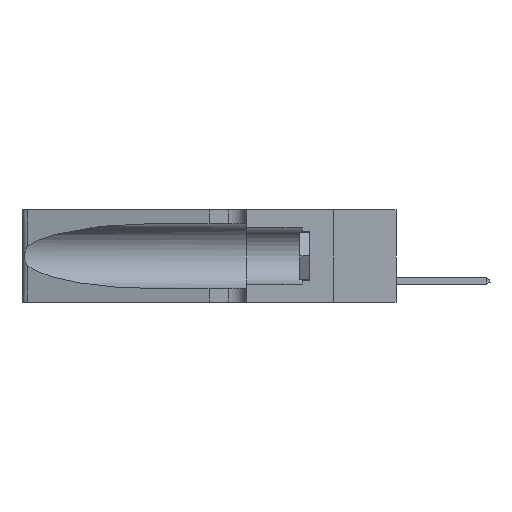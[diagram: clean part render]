
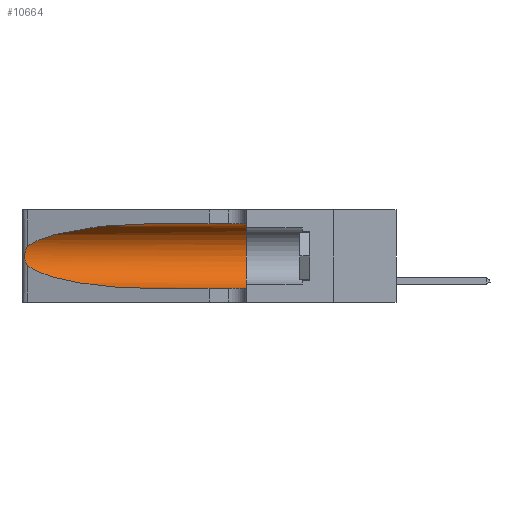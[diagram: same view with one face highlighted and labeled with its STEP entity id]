
A CAD part, left-side view. The second image highlights one B-rep face of the part: STEP entity #10664.
In plain terms, the highlighted cylindrical face has radius 3.308 mm (diameter 6.617 mm), a partial arc.
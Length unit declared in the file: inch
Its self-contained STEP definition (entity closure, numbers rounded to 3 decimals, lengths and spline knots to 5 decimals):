
#4 = CARTESIAN_POINT ( 'NONE',  ( 0.1305, 0.35, 0.31525 ) ) ;
#23 = ORIENTED_EDGE ( 'NONE', *, *, #19158, .F. ) ;
#494 = CARTESIAN_POINT ( 'NONE',  ( 0.25555, 1.22993, 0.14849 ) ) ;
#728 = CARTESIAN_POINT ( 'NONE',  ( 0.18966, 0.96281, 0.05475 ) ) ;
#735 = CARTESIAN_POINT ( 'NONE',  ( 0.25487, 1.22718, 0.22369 ) ) ;
#1291 = DIRECTION ( 'NONE',  ( 0., -1., 0. ) ) ;
#1367 = AXIS2_PLACEMENT_3D ( 'NONE', #32556, #1291, #26429 ) ;
#1654 = LINE ( 'NONE', #19210, #11016 ) ;
#2381 = DIRECTION ( 'NONE',  ( 0., 1., 0. ) ) ;
#3594 =( BOUNDED_CURVE ( )  B_SPLINE_CURVE ( 3, ( #3757, #31983, #19567, #735 ),
 .UNSPECIFIED., .F., .F. ) 
 B_SPLINE_CURVE_WITH_KNOTS ( ( 4, 4 ),
 ( 1.5708, 2.84003 ),
 .UNSPECIFIED. ) 
 CURVE ( )  GEOMETRIC_REPRESENTATION_ITEM ( )  RATIONAL_B_SPLINE_CURVE ( ( 1., 0.87, 0.87, 1. ) ) 
 REPRESENTATION_ITEM ( '' )  );
#3757 = CARTESIAN_POINT ( 'NONE',  ( 0.1305, 0.72297, 0.31525 ) ) ;
#5365 = CARTESIAN_POINT ( 'NONE',  ( 0.26075, 1.23896, 0.19203 ) ) ;
#5766 = CARTESIAN_POINT ( 'NONE',  ( 0.26017, 1.23833, 0.17102 ) ) ;
#6132 = B_SPLINE_CURVE_WITH_KNOTS ( 'NONE', 3,
 ( #21737, #19653, #10298, #34682, #15936, #33316, #5365, #36600, #5766, #25374, #19859, #9836, #494, #10801 ),
 .UNSPECIFIED., .F., .F.,
 ( 4, 2, 2, 2, 2, 2, 4 ),
 ( 0., 0.00027, 0.00053, 0.00107, 0.0016, 0.00187, 0.00214 ),
 .UNSPECIFIED. ) ;
#6806 = CARTESIAN_POINT ( 'NONE',  ( 0.1305, 0.72297, 0.31525 ) ) ;
#6896 = CARTESIAN_POINT ( 'NONE',  ( 0.2373, 1.15595, 0.08982 ) ) ;
#7264 = CARTESIAN_POINT ( 'NONE',  ( 0.25487, 1.22718, 0.14631 ) ) ;
#8649 =( BOUNDED_CURVE ( )  B_SPLINE_CURVE ( 3, ( #38559, #6896, #728, #13506 ),
 .UNSPECIFIED., .F., .T. ) 
 B_SPLINE_CURVE_WITH_KNOTS ( ( 4, 4 ),
 ( 3.44316, 4.71239 ),
 .UNSPECIFIED. ) 
 CURVE ( )  GEOMETRIC_REPRESENTATION_ITEM ( )  RATIONAL_B_SPLINE_CURVE ( ( 1., 0.87, 0.87, 1. ) ) 
 REPRESENTATION_ITEM ( '' )  );
#9836 = CARTESIAN_POINT ( 'NONE',  ( 0.25639, 1.23186, 0.15144 ) ) ;
#10298 = CARTESIAN_POINT ( 'NONE',  ( 0.25639, 1.23184, 0.21858 ) ) ;
#10318 = EDGE_CURVE ( 'NONE', #38061, #22144, #28566, .T. ) ;
#10664 = ADVANCED_FACE ( 'NONE', ( #22173 ), #20757, .F. ) ;
#10801 = CARTESIAN_POINT ( 'NONE',  ( 0.25487, 1.22718, 0.14631 ) ) ;
#11016 = VECTOR ( 'NONE', #28136, 39.37008 ) ;
#12293 = DIRECTION ( 'NONE',  ( 0., -1., 0. ) ) ;
#13506 = CARTESIAN_POINT ( 'NONE',  ( 0.1305, 0.72297, 0.05475 ) ) ;
#15395 = VERTEX_POINT ( 'NONE', #31960 ) ;
#15936 = CARTESIAN_POINT ( 'NONE',  ( 0.25854, 1.2359, 0.20912 ) ) ;
#18486 = VERTEX_POINT ( 'NONE', #24417 ) ;
#19158 = EDGE_CURVE ( 'NONE', #23002, #38061, #21104, .T. ) ;
#19210 = CARTESIAN_POINT ( 'NONE',  ( 0.1305, 1.61858, 0.05475 ) ) ;
#19511 = VERTEX_POINT ( 'NONE', #7264 ) ;
#19567 = CARTESIAN_POINT ( 'NONE',  ( 0.2373, 1.15595, 0.28018 ) ) ;
#19653 = CARTESIAN_POINT ( 'NONE',  ( 0.25555, 1.22994, 0.2215 ) ) ;
#19859 = CARTESIAN_POINT ( 'NONE',  ( 0.25789, 1.23486, 0.15765 ) ) ;
#20037 = CARTESIAN_POINT ( 'NONE',  ( 0.1305, 0.35, 0.05475 ) ) ;
#20651 = EDGE_CURVE ( 'NONE', #19511, #15395, #8649, .T. ) ;
#20757 = CYLINDRICAL_SURFACE ( 'NONE', #1367, 0.13025 ) ;
#21104 = LINE ( 'NONE', #24922, #38686 ) ;
#21737 = CARTESIAN_POINT ( 'NONE',  ( 0.25487, 1.22718, 0.22369 ) ) ;
#22144 = VERTEX_POINT ( 'NONE', #20037 ) ;
#22173 = FACE_OUTER_BOUND ( 'NONE', #33505, .T. ) ;
#23002 = VERTEX_POINT ( 'NONE', #6806 ) ;
#23127 = ORIENTED_EDGE ( 'NONE', *, *, #25443, .T. ) ;
#24417 = CARTESIAN_POINT ( 'NONE',  ( 0.25487, 1.22718, 0.22369 ) ) ;
#24922 = CARTESIAN_POINT ( 'NONE',  ( 0.1305, 1.61858, 0.31525 ) ) ;
#25374 = CARTESIAN_POINT ( 'NONE',  ( 0.25856, 1.23593, 0.16098 ) ) ;
#25443 = EDGE_CURVE ( 'NONE', #15395, #22144, #1654, .T. ) ;
#26429 = DIRECTION ( 'NONE',  ( 0., 0., -1. ) ) ;
#28051 = CARTESIAN_POINT ( 'NONE',  ( 0.1305, 0.35, 0.185 ) ) ;
#28136 = DIRECTION ( 'NONE',  ( 0., -1., 0. ) ) ;
#28566 = CIRCLE ( 'NONE', #37117, 0.13025 ) ;
#28799 = ORIENTED_EDGE ( 'NONE', *, *, #10318, .F. ) ;
#28817 = ORIENTED_EDGE ( 'NONE', *, *, #20651, .T. ) ;
#31021 = ORIENTED_EDGE ( 'NONE', *, *, #31098, .T. ) ;
#31098 = EDGE_CURVE ( 'NONE', #18486, #19511, #6132, .T. ) ;
#31960 = CARTESIAN_POINT ( 'NONE',  ( 0.1305, 0.72297, 0.05475 ) ) ;
#31983 = CARTESIAN_POINT ( 'NONE',  ( 0.18966, 0.96281, 0.31525 ) ) ;
#32556 = CARTESIAN_POINT ( 'NONE',  ( 0.1305, 1.61858, 0.185 ) ) ;
#33316 = CARTESIAN_POINT ( 'NONE',  ( 0.26018, 1.23835, 0.19895 ) ) ;
#33505 = EDGE_LOOP ( 'NONE', ( #35954, #31021, #28817, #23127, #28799, #23 ) ) ;
#34682 = CARTESIAN_POINT ( 'NONE',  ( 0.25787, 1.23484, 0.2124 ) ) ;
#35954 = ORIENTED_EDGE ( 'NONE', *, *, #37041, .T. ) ;
#36600 = CARTESIAN_POINT ( 'NONE',  ( 0.26075, 1.23896, 0.178 ) ) ;
#36952 = DIRECTION ( 'NONE',  ( 0., 0., 1. ) ) ;
#37041 = EDGE_CURVE ( 'NONE', #23002, #18486, #3594, .T. ) ;
#37117 = AXIS2_PLACEMENT_3D ( 'NONE', #28051, #2381, #36952 ) ;
#38061 = VERTEX_POINT ( 'NONE', #4 ) ;
#38559 = CARTESIAN_POINT ( 'NONE',  ( 0.25487, 1.22718, 0.14631 ) ) ;
#38686 = VECTOR ( 'NONE', #12293, 39.37008 ) ;
